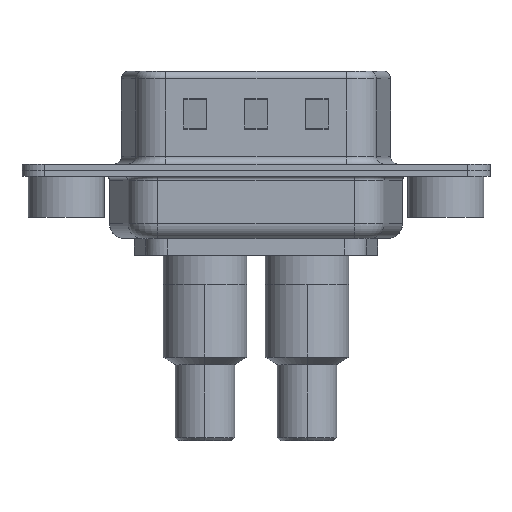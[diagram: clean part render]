
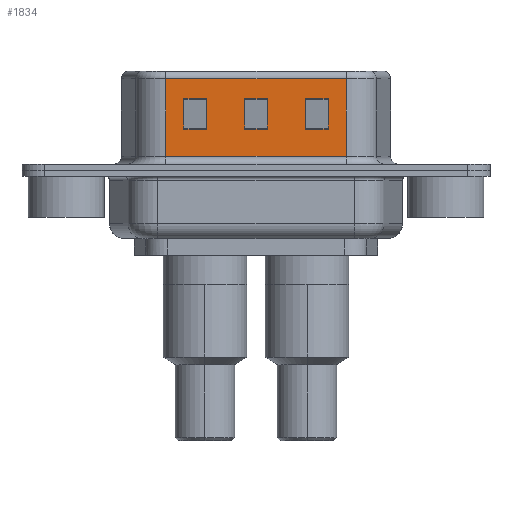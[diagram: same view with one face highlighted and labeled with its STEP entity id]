
A CAD part, front view. The second image highlights one B-rep face of the part: STEP entity #1834.
In plain terms, the highlighted planar face has unit normal (0, -1, 0).
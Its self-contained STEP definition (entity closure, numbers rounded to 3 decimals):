
#6 = EDGE_CURVE ( 'NONE', #8207, #14231, #274, .T. ) ;
#274 = LINE ( 'NONE', #21511, #13393 ) ;
#431 = ORIENTED_EDGE ( 'NONE', *, *, #871, .T. ) ;
#773 = VECTOR ( 'NONE', #1388, 1000. ) ;
#871 = EDGE_CURVE ( 'NONE', #11804, #12437, #13120, .T. ) ;
#908 = CARTESIAN_POINT ( 'NONE',  ( 6.55, -4.58, 6.02 ) ) ;
#1388 = DIRECTION ( 'NONE',  ( 0., 0., -1. ) ) ;
#1411 = ORIENTED_EDGE ( 'NONE', *, *, #17369, .F. ) ;
#1571 = CARTESIAN_POINT ( 'NONE',  ( 22.45, -4.58, 4.705 ) ) ;
#1687 = CARTESIAN_POINT ( 'NONE',  ( 22.45, -4.58, 2.705 ) ) ;
#1834 = ADVANCED_FACE ( 'NONE', ( #2821, #20506, #16244, #20021 ), #20811, .F. ) ;
#2388 = ORIENTED_EDGE ( 'NONE', *, *, #4382, .T. ) ;
#2427 = VECTOR ( 'NONE', #6082, 1000. ) ;
#2594 = VERTEX_POINT ( 'NONE', #5630 ) ;
#2684 = ORIENTED_EDGE ( 'NONE', *, *, #9132, .T. ) ;
#2692 = CARTESIAN_POINT ( 'NONE',  ( 7.75, -4.58, 6.52 ) ) ;
#2770 = CARTESIAN_POINT ( 'NONE',  ( 15.75, -4.58, 6.52 ) ) ;
#2821 = FACE_BOUND ( 'NONE', #14352, .T. ) ;
#3068 = ORIENTED_EDGE ( 'NONE', *, *, #13212, .T. ) ;
#3082 = DIRECTION ( 'NONE',  ( -1., 0., 0. ) ) ;
#3133 = CARTESIAN_POINT ( 'NONE',  ( 9.25, -4.58, 4.705 ) ) ;
#3575 = VECTOR ( 'NONE', #6946, 1000. ) ;
#3741 = CARTESIAN_POINT ( 'NONE',  ( 18.45, -4.58, 6.02 ) ) ;
#3846 = CARTESIAN_POINT ( 'NONE',  ( 11.75, -4.58, 4.705 ) ) ;
#4382 = EDGE_CURVE ( 'NONE', #12437, #9969, #5993, .T. ) ;
#4910 = DIRECTION ( 'NONE',  ( 0., 0., 1. ) ) ;
#5294 = ORIENTED_EDGE ( 'NONE', *, *, #17804, .T. ) ;
#5630 = CARTESIAN_POINT ( 'NONE',  ( 18.45, -4.58, 0.9 ) ) ;
#5664 = CARTESIAN_POINT ( 'NONE',  ( 18.45, -4.58, 6.52 ) ) ;
#5810 = ORIENTED_EDGE ( 'NONE', *, *, #10299, .T. ) ;
#5993 = LINE ( 'NONE', #17459, #14295 ) ;
#6042 = CARTESIAN_POINT ( 'NONE',  ( 18.45, -4.58, 6.02 ) ) ;
#6045 = DIRECTION ( 'NONE',  ( -1., 0., 0. ) ) ;
#6082 = DIRECTION ( 'NONE',  ( 0., 0., -1. ) ) ;
#6436 = CARTESIAN_POINT ( 'NONE',  ( 17.25, -4.58, 4.705 ) ) ;
#6458 = LINE ( 'NONE', #3741, #15305 ) ;
#6734 = CARTESIAN_POINT ( 'NONE',  ( 9.25, -4.58, 2.705 ) ) ;
#6935 = EDGE_CURVE ( 'NONE', #9969, #17587, #13707, .T. ) ;
#6946 = DIRECTION ( 'NONE',  ( -1., 0., 0. ) ) ;
#7215 = VERTEX_POINT ( 'NONE', #6042 ) ;
#7337 = CARTESIAN_POINT ( 'NONE',  ( 18.45, -4.58, 4.705 ) ) ;
#7355 = VECTOR ( 'NONE', #11931, 1000. ) ;
#7883 = ORIENTED_EDGE ( 'NONE', *, *, #10781, .T. ) ;
#8179 = LINE ( 'NONE', #11444, #11565 ) ;
#8207 = VERTEX_POINT ( 'NONE', #19918 ) ;
#8787 = VECTOR ( 'NONE', #4910, 1000. ) ;
#8913 = LINE ( 'NONE', #13283, #773 ) ;
#9132 = EDGE_CURVE ( 'NONE', #14231, #9431, #8179, .T. ) ;
#9431 = VERTEX_POINT ( 'NONE', #20402 ) ;
#9619 = CARTESIAN_POINT ( 'NONE',  ( 17.25, -4.58, 2.705 ) ) ;
#9753 = VERTEX_POINT ( 'NONE', #21138 ) ;
#9790 = ORIENTED_EDGE ( 'NONE', *, *, #12931, .T. ) ;
#9897 = VECTOR ( 'NONE', #10201, 1000. ) ;
#9969 = VERTEX_POINT ( 'NONE', #10166 ) ;
#10166 = CARTESIAN_POINT ( 'NONE',  ( 7.75, -4.58, 2.705 ) ) ;
#10201 = DIRECTION ( 'NONE',  ( 1., 0., 0. ) ) ;
#10299 = EDGE_CURVE ( 'NONE', #17587, #11804, #11825, .T. ) ;
#10453 = VERTEX_POINT ( 'NONE', #3846 ) ;
#10714 = VECTOR ( 'NONE', #14432, 1000. ) ;
#10781 = EDGE_CURVE ( 'NONE', #13634, #9753, #8913, .T. ) ;
#10922 = AXIS2_PLACEMENT_3D ( 'NONE', #5664, #19259, #16950 ) ;
#11014 = ORIENTED_EDGE ( 'NONE', *, *, #18778, .T. ) ;
#11444 = CARTESIAN_POINT ( 'NONE',  ( 18.45, -4.58, 2.705 ) ) ;
#11565 = VECTOR ( 'NONE', #3082, 1000. ) ;
#11673 = EDGE_CURVE ( 'NONE', #20639, #13653, #19943, .T. ) ;
#11720 = VECTOR ( 'NONE', #17226, 1000. ) ;
#11804 = VERTEX_POINT ( 'NONE', #3133 ) ;
#11825 = LINE ( 'NONE', #21730, #7355 ) ;
#11931 = DIRECTION ( 'NONE',  ( 1., 0., 0. ) ) ;
#12138 = DIRECTION ( 'NONE',  ( -1., 0., 0. ) ) ;
#12336 = CARTESIAN_POINT ( 'NONE',  ( 15.75, -4.58, 2.705 ) ) ;
#12437 = VERTEX_POINT ( 'NONE', #6734 ) ;
#12513 = LINE ( 'NONE', #1687, #3575 ) ;
#12520 = EDGE_CURVE ( 'NONE', #13653, #14392, #12513, .T. ) ;
#12869 = CARTESIAN_POINT ( 'NONE',  ( 17.25, -4.58, 6.52 ) ) ;
#12931 = EDGE_CURVE ( 'NONE', #14392, #19718, #15082, .T. ) ;
#13120 = LINE ( 'NONE', #18339, #17423 ) ;
#13212 = EDGE_CURVE ( 'NONE', #19718, #20639, #18625, .T. ) ;
#13283 = CARTESIAN_POINT ( 'NONE',  ( 6.55, -4.58, 6.52 ) ) ;
#13393 = VECTOR ( 'NONE', #17543, 1000. ) ;
#13422 = ORIENTED_EDGE ( 'NONE', *, *, #14303, .T. ) ;
#13441 = EDGE_CURVE ( 'NONE', #10453, #8207, #16096, .T. ) ;
#13634 = VERTEX_POINT ( 'NONE', #908 ) ;
#13653 = VERTEX_POINT ( 'NONE', #9619 ) ;
#13677 = ORIENTED_EDGE ( 'NONE', *, *, #11673, .T. ) ;
#13707 = LINE ( 'NONE', #2692, #8787 ) ;
#14012 = VECTOR ( 'NONE', #21108, 1000. ) ;
#14026 = VECTOR ( 'NONE', #16371, 1000. ) ;
#14173 = EDGE_LOOP ( 'NONE', ( #18626, #15498, #2684, #5294 ) ) ;
#14231 = VERTEX_POINT ( 'NONE', #18554 ) ;
#14295 = VECTOR ( 'NONE', #6045, 1000. ) ;
#14303 = EDGE_CURVE ( 'NONE', #7215, #13634, #6458, .T. ) ;
#14352 = EDGE_LOOP ( 'NONE', ( #431, #2388, #20047, #5810 ) ) ;
#14392 = VERTEX_POINT ( 'NONE', #12336 ) ;
#14432 = DIRECTION ( 'NONE',  ( 0., 0., 1. ) ) ;
#14493 = DIRECTION ( 'NONE',  ( 0., 0., -1. ) ) ;
#14562 = LINE ( 'NONE', #21143, #10714 ) ;
#14885 = DIRECTION ( 'NONE',  ( 0., 0., -1. ) ) ;
#15082 = LINE ( 'NONE', #2770, #14012 ) ;
#15203 = CARTESIAN_POINT ( 'NONE',  ( 15.75, -4.58, 4.705 ) ) ;
#15305 = VECTOR ( 'NONE', #12138, 1000. ) ;
#15498 = ORIENTED_EDGE ( 'NONE', *, *, #6, .T. ) ;
#15662 = VECTOR ( 'NONE', #14493, 1000. ) ;
#15899 = LINE ( 'NONE', #16034, #2427 ) ;
#16034 = CARTESIAN_POINT ( 'NONE',  ( 18.45, -4.58, 6.52 ) ) ;
#16096 = LINE ( 'NONE', #7337, #11720 ) ;
#16244 = FACE_BOUND ( 'NONE', #14173, .T. ) ;
#16371 = DIRECTION ( 'NONE',  ( 1., 0., 0. ) ) ;
#16950 = DIRECTION ( 'NONE',  ( 0., 0., 1. ) ) ;
#17226 = DIRECTION ( 'NONE',  ( 1., 0., 0. ) ) ;
#17369 = EDGE_CURVE ( 'NONE', #7215, #2594, #15899, .T. ) ;
#17423 = VECTOR ( 'NONE', #14885, 1000. ) ;
#17459 = CARTESIAN_POINT ( 'NONE',  ( 14.45, -4.58, 2.705 ) ) ;
#17543 = DIRECTION ( 'NONE',  ( 0., 0., -1. ) ) ;
#17587 = VERTEX_POINT ( 'NONE', #19009 ) ;
#17804 = EDGE_CURVE ( 'NONE', #9431, #10453, #14562, .T. ) ;
#17955 = EDGE_LOOP ( 'NONE', ( #13677, #20343, #9790, #3068 ) ) ;
#18339 = CARTESIAN_POINT ( 'NONE',  ( 9.25, -4.58, 6.52 ) ) ;
#18554 = CARTESIAN_POINT ( 'NONE',  ( 13.25, -4.58, 2.705 ) ) ;
#18625 = LINE ( 'NONE', #1571, #9897 ) ;
#18626 = ORIENTED_EDGE ( 'NONE', *, *, #13441, .T. ) ;
#18778 = EDGE_CURVE ( 'NONE', #9753, #2594, #21708, .T. ) ;
#19009 = CARTESIAN_POINT ( 'NONE',  ( 7.75, -4.58, 4.705 ) ) ;
#19259 = DIRECTION ( 'NONE',  ( 0., 1., 0. ) ) ;
#19718 = VERTEX_POINT ( 'NONE', #15203 ) ;
#19918 = CARTESIAN_POINT ( 'NONE',  ( 13.25, -4.58, 4.705 ) ) ;
#19943 = LINE ( 'NONE', #12869, #15662 ) ;
#20021 = FACE_OUTER_BOUND ( 'NONE', #21441, .T. ) ;
#20047 = ORIENTED_EDGE ( 'NONE', *, *, #6935, .T. ) ;
#20343 = ORIENTED_EDGE ( 'NONE', *, *, #12520, .T. ) ;
#20402 = CARTESIAN_POINT ( 'NONE',  ( 11.75, -4.58, 2.705 ) ) ;
#20506 = FACE_BOUND ( 'NONE', #17955, .T. ) ;
#20639 = VERTEX_POINT ( 'NONE', #6436 ) ;
#20811 = PLANE ( 'NONE',  #10922 ) ;
#21108 = DIRECTION ( 'NONE',  ( 0., 0., 1. ) ) ;
#21138 = CARTESIAN_POINT ( 'NONE',  ( 6.55, -4.58, 0.9 ) ) ;
#21143 = CARTESIAN_POINT ( 'NONE',  ( 11.75, -4.58, 6.52 ) ) ;
#21188 = CARTESIAN_POINT ( 'NONE',  ( 18.45, -4.58, 0.9 ) ) ;
#21441 = EDGE_LOOP ( 'NONE', ( #1411, #13422, #7883, #11014 ) ) ;
#21511 = CARTESIAN_POINT ( 'NONE',  ( 13.25, -4.58, 6.52 ) ) ;
#21708 = LINE ( 'NONE', #21188, #14026 ) ;
#21730 = CARTESIAN_POINT ( 'NONE',  ( 14.45, -4.58, 4.705 ) ) ;
